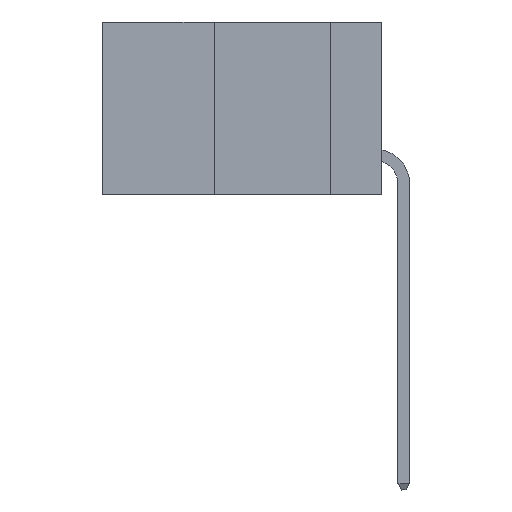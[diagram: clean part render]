
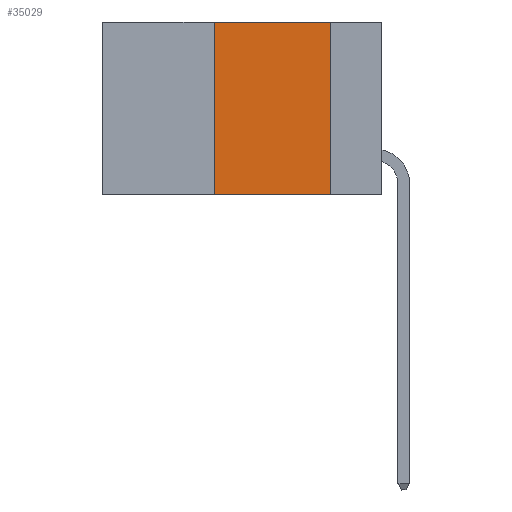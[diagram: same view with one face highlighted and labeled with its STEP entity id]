
A CAD part, left-side view. The second image highlights one B-rep face of the part: STEP entity #35029.
In plain terms, the highlighted planar face has unit normal (-1, 0, 0).
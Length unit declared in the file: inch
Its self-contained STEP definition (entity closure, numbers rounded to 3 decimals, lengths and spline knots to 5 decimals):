
#3261 = FACE_OUTER_BOUND ( 'NONE', #19606, .T. ) ;
#3370 = CARTESIAN_POINT ( 'NONE',  ( 0., 0.36, -0.37 ) ) ;
#3675 = VECTOR ( 'NONE', #28289, 39.37008 ) ;
#3754 = AXIS2_PLACEMENT_3D ( 'NONE', #39558, #23939, #8488 ) ;
#5455 = CARTESIAN_POINT ( 'NONE',  ( 0., 0.6, -0.37 ) ) ;
#5905 = VERTEX_POINT ( 'NONE', #31234 ) ;
#8154 = LINE ( 'NONE', #5455, #15497 ) ;
#8213 = ORIENTED_EDGE ( 'NONE', *, *, #16291, .T. ) ;
#8488 = DIRECTION ( 'NONE',  ( 0., 0., -1. ) ) ;
#9976 = LINE ( 'NONE', #18337, #3675 ) ;
#10446 = CARTESIAN_POINT ( 'NONE',  ( 0., 0.11, 0. ) ) ;
#11821 = DIRECTION ( 'NONE',  ( 0., -1., 0. ) ) ;
#13241 = ORIENTED_EDGE ( 'NONE', *, *, #30135, .F. ) ;
#14350 = DIRECTION ( 'NONE',  ( 0., -1., 0. ) ) ;
#15497 = VECTOR ( 'NONE', #11821, 39.37008 ) ;
#15946 = VERTEX_POINT ( 'NONE', #34597 ) ;
#16291 = EDGE_CURVE ( 'NONE', #28430, #19303, #8154, .T. ) ;
#16902 = EDGE_CURVE ( 'NONE', #28430, #5905, #9976, .T. ) ;
#18337 = CARTESIAN_POINT ( 'NONE',  ( 0., 0.36, 0. ) ) ;
#19303 = VERTEX_POINT ( 'NONE', #37430 ) ;
#19606 = EDGE_LOOP ( 'NONE', ( #38917, #13241, #39083, #8213 ) ) ;
#21933 = VECTOR ( 'NONE', #25506, 39.37008 ) ;
#23939 = DIRECTION ( 'NONE',  ( 1., 0., 0. ) ) ;
#25506 = DIRECTION ( 'NONE',  ( 0., 0., -1. ) ) ;
#28289 = DIRECTION ( 'NONE',  ( 0., 0., 1. ) ) ;
#28430 = VERTEX_POINT ( 'NONE', #3370 ) ;
#29710 = VECTOR ( 'NONE', #14350, 39.37008 ) ;
#30099 = LINE ( 'NONE', #10446, #21933 ) ;
#30135 = EDGE_CURVE ( 'NONE', #5905, #15946, #37807, .T. ) ;
#31234 = CARTESIAN_POINT ( 'NONE',  ( 0., 0.36, 0. ) ) ;
#31723 = EDGE_CURVE ( 'NONE', #15946, #19303, #30099, .T. ) ;
#34597 = CARTESIAN_POINT ( 'NONE',  ( 0., 0.11, 0. ) ) ;
#35029 = ADVANCED_FACE ( 'NONE', ( #3261 ), #36098, .F. ) ;
#36098 = PLANE ( 'NONE',  #3754 ) ;
#37430 = CARTESIAN_POINT ( 'NONE',  ( 0., 0.11, -0.37 ) ) ;
#37807 = LINE ( 'NONE', #39167, #29710 ) ;
#38917 = ORIENTED_EDGE ( 'NONE', *, *, #31723, .F. ) ;
#39083 = ORIENTED_EDGE ( 'NONE', *, *, #16902, .F. ) ;
#39167 = CARTESIAN_POINT ( 'NONE',  ( 0., 0.6, 0. ) ) ;
#39558 = CARTESIAN_POINT ( 'NONE',  ( 0., 0.6, 0. ) ) ;
